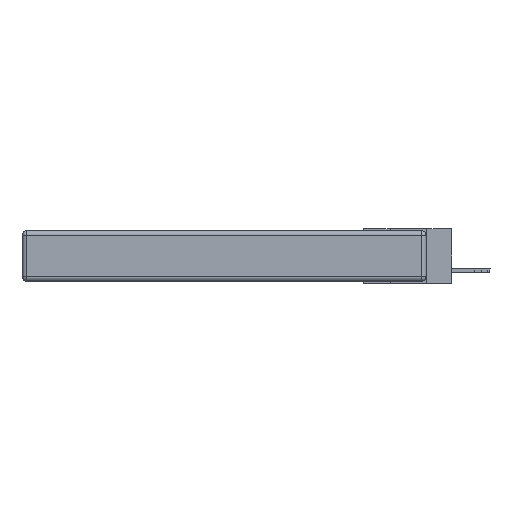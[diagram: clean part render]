
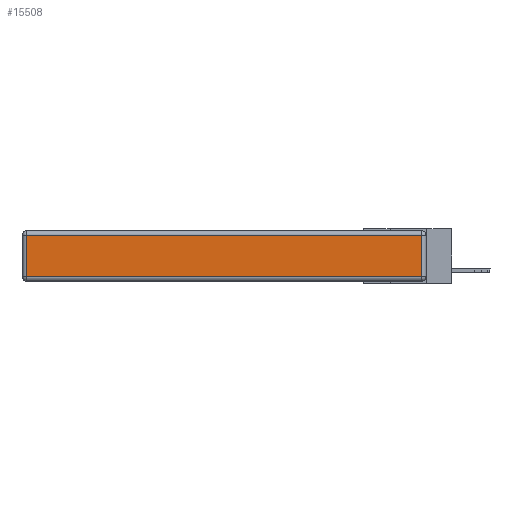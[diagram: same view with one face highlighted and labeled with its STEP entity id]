
A CAD part, left-side view. The second image highlights one B-rep face of the part: STEP entity #15508.
In plain terms, the highlighted planar face has unit normal (-1, 0, 0).
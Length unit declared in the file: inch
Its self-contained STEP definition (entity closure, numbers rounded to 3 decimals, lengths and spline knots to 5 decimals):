
#209 = CARTESIAN_POINT ( 'NONE',  ( 0., 0., -0.313 ) ) ;
#818 = VERTEX_POINT ( 'NONE', #12347 ) ;
#1004 = CARTESIAN_POINT ( 'NONE',  ( 0., 2.72, -0.343 ) ) ;
#1494 = LINE ( 'NONE', #1004, #21149 ) ;
#1556 = FACE_OUTER_BOUND ( 'NONE', #7192, .T. ) ;
#1632 = DIRECTION ( 'NONE',  ( 0., 1., 0. ) ) ;
#2393 = DIRECTION ( 'NONE',  ( 0., -1., 0. ) ) ;
#3223 = VECTOR ( 'NONE', #14101, 39.37008 ) ;
#3376 = DIRECTION ( 'NONE',  ( 0., 0., 1. ) ) ;
#3421 = CARTESIAN_POINT ( 'NONE',  ( 0., 0.03, -0.313 ) ) ;
#5226 = VECTOR ( 'NONE', #2393, 39.37008 ) ;
#5675 = CARTESIAN_POINT ( 'NONE',  ( 0., 0.03, -0.343 ) ) ;
#5937 = LINE ( 'NONE', #17513, #25280 ) ;
#6564 = AXIS2_PLACEMENT_3D ( 'NONE', #19254, #19168, #3376 ) ;
#7192 = EDGE_LOOP ( 'NONE', ( #23971, #14790, #9691, #18592 ) ) ;
#7303 = PLANE ( 'NONE',  #6564 ) ;
#7574 = EDGE_CURVE ( 'NONE', #11289, #16149, #8471, .T. ) ;
#8336 = EDGE_CURVE ( 'NONE', #16149, #21468, #5937, .T. ) ;
#8471 = LINE ( 'NONE', #5675, #3223 ) ;
#9691 = ORIENTED_EDGE ( 'NONE', *, *, #8336, .T. ) ;
#11289 = VERTEX_POINT ( 'NONE', #3421 ) ;
#12347 = CARTESIAN_POINT ( 'NONE',  ( 0., 2.72, -0.313 ) ) ;
#12489 = CARTESIAN_POINT ( 'NONE',  ( 0., 2.72, -0.03 ) ) ;
#12978 = EDGE_CURVE ( 'NONE', #818, #11289, #22139, .T. ) ;
#14101 = DIRECTION ( 'NONE',  ( 0., 0., 1. ) ) ;
#14408 = EDGE_CURVE ( 'NONE', #21468, #818, #1494, .T. ) ;
#14776 = CARTESIAN_POINT ( 'NONE',  ( 0., 0.03, -0.03 ) ) ;
#14790 = ORIENTED_EDGE ( 'NONE', *, *, #7574, .T. ) ;
#15508 = ADVANCED_FACE ( 'NONE', ( #1556 ), #7303, .T. ) ;
#16149 = VERTEX_POINT ( 'NONE', #14776 ) ;
#17513 = CARTESIAN_POINT ( 'NONE',  ( 0., 2.75, -0.03 ) ) ;
#18592 = ORIENTED_EDGE ( 'NONE', *, *, #14408, .T. ) ;
#19168 = DIRECTION ( 'NONE',  ( -1., 0., 0. ) ) ;
#19254 = CARTESIAN_POINT ( 'NONE',  ( 0., 0., -0.343 ) ) ;
#20603 = DIRECTION ( 'NONE',  ( 0., 0., -1. ) ) ;
#21149 = VECTOR ( 'NONE', #20603, 39.37008 ) ;
#21468 = VERTEX_POINT ( 'NONE', #12489 ) ;
#22139 = LINE ( 'NONE', #209, #5226 ) ;
#23971 = ORIENTED_EDGE ( 'NONE', *, *, #12978, .T. ) ;
#25280 = VECTOR ( 'NONE', #1632, 39.37008 ) ;
